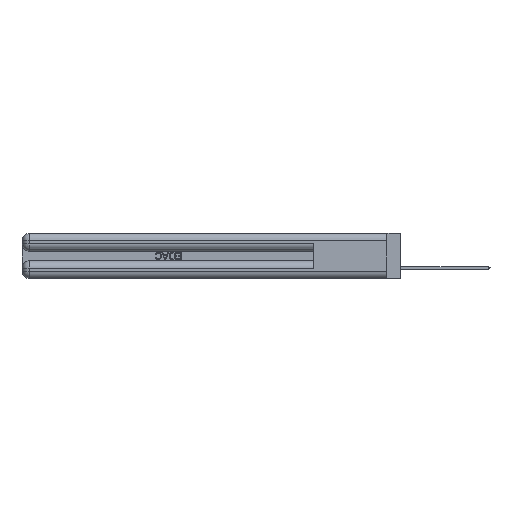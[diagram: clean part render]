
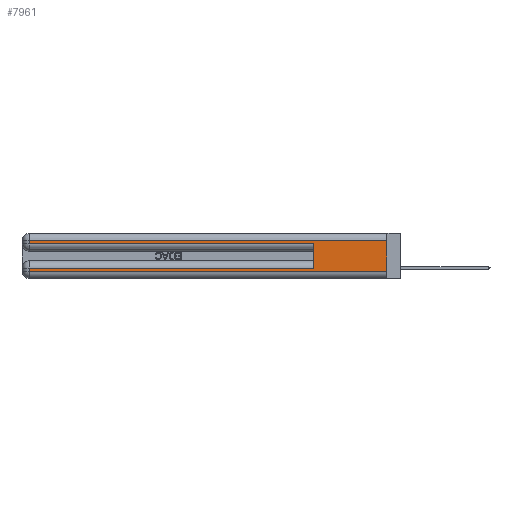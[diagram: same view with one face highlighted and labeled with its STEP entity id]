
A CAD part, left-side view. The second image highlights one B-rep face of the part: STEP entity #7961.
In plain terms, the highlighted planar face has unit normal (-1, 0, 0).
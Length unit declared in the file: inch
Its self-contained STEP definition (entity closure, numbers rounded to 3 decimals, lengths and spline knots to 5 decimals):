
#307 = VERTEX_POINT ( 'NONE', #35947 ) ;
#686 = VECTOR ( 'NONE', #15018, 39.37008 ) ;
#875 = DIRECTION ( 'NONE',  ( 0., 0., 1. ) ) ;
#906 = VERTEX_POINT ( 'NONE', #15071 ) ;
#1614 = CARTESIAN_POINT ( 'NONE',  ( 0., 0.6, 0.145 ) ) ;
#2064 = ORIENTED_EDGE ( 'NONE', *, *, #6542, .T. ) ;
#2390 = VERTEX_POINT ( 'NONE', #4002 ) ;
#2980 = CARTESIAN_POINT ( 'NONE',  ( 0., 0., 0.285 ) ) ;
#4002 = CARTESIAN_POINT ( 'NONE',  ( 0., 2.94, 0.06 ) ) ;
#6542 = EDGE_CURVE ( 'NONE', #906, #47553, #38171, .T. ) ;
#6852 = EDGE_CURVE ( 'NONE', #36797, #906, #35627, .T. ) ;
#7961 = ADVANCED_FACE ( 'NONE', ( #22028 ), #9699, .F. ) ;
#8759 = CARTESIAN_POINT ( 'NONE',  ( 0., 0., 0.37 ) ) ;
#9699 = PLANE ( 'NONE',  #32679 ) ;
#9749 = ORIENTED_EDGE ( 'NONE', *, *, #37751, .F. ) ;
#9821 = VERTEX_POINT ( 'NONE', #17732 ) ;
#11307 = ORIENTED_EDGE ( 'NONE', *, *, #6852, .T. ) ;
#11469 = CARTESIAN_POINT ( 'NONE',  ( 0., 0., 0.06 ) ) ;
#12761 = LINE ( 'NONE', #8759, #19110 ) ;
#14508 = CARTESIAN_POINT ( 'NONE',  ( 0., 0., 0.31 ) ) ;
#15018 = DIRECTION ( 'NONE',  ( 0., 0., -1. ) ) ;
#15071 = CARTESIAN_POINT ( 'NONE',  ( 0., 2.94, 0.285 ) ) ;
#15476 = VECTOR ( 'NONE', #30989, 39.37008 ) ;
#16840 = ORIENTED_EDGE ( 'NONE', *, *, #33556, .T. ) ;
#16868 = EDGE_CURVE ( 'NONE', #307, #2390, #34817, .T. ) ;
#16873 = DIRECTION ( 'NONE',  ( 0., 0., -1. ) ) ;
#16973 = ORIENTED_EDGE ( 'NONE', *, *, #19357, .T. ) ;
#17632 = EDGE_LOOP ( 'NONE', ( #40382, #16973, #11307, #2064, #9749, #35689, #32387, #16840 ) ) ;
#17732 = CARTESIAN_POINT ( 'NONE',  ( 0., 0., 0.06 ) ) ;
#17960 = CARTESIAN_POINT ( 'NONE',  ( 0., 0.6, 0.085 ) ) ;
#19110 = VECTOR ( 'NONE', #16873, 39.37008 ) ;
#19357 = EDGE_CURVE ( 'NONE', #49574, #36797, #33866, .T. ) ;
#19850 = DIRECTION ( 'NONE',  ( 0., -1., 0. ) ) ;
#20785 = CARTESIAN_POINT ( 'NONE',  ( 0., 2.94, 0.37 ) ) ;
#21712 = DIRECTION ( 'NONE',  ( 0., 0., -1. ) ) ;
#21976 = LINE ( 'NONE', #1614, #29412 ) ;
#22028 = FACE_OUTER_BOUND ( 'NONE', #17632, .T. ) ;
#22784 = VECTOR ( 'NONE', #34287, 39.37008 ) ;
#26971 = VECTOR ( 'NONE', #43122, 39.37008 ) ;
#27278 = CARTESIAN_POINT ( 'NONE',  ( 0., 0., 0.31 ) ) ;
#29412 = VECTOR ( 'NONE', #875, 39.37008 ) ;
#29976 = CARTESIAN_POINT ( 'NONE',  ( 0., 0., 0.37 ) ) ;
#30989 = DIRECTION ( 'NONE',  ( 0., -1., 0. ) ) ;
#32387 = ORIENTED_EDGE ( 'NONE', *, *, #16868, .T. ) ;
#32657 = VERTEX_POINT ( 'NONE', #17960 ) ;
#32679 = AXIS2_PLACEMENT_3D ( 'NONE', #29976, #38669, #21712 ) ;
#32737 = VECTOR ( 'NONE', #19850, 39.37008 ) ;
#33424 = LINE ( 'NONE', #50688, #22784 ) ;
#33443 = CARTESIAN_POINT ( 'NONE',  ( 0., 0.6, 0.285 ) ) ;
#33556 = EDGE_CURVE ( 'NONE', #2390, #9821, #42250, .T. ) ;
#33866 = LINE ( 'NONE', #14508, #26971 ) ;
#34287 = DIRECTION ( 'NONE',  ( 0., 1., 0. ) ) ;
#34355 = DIRECTION ( 'NONE',  ( 0., 0., -1. ) ) ;
#34817 = LINE ( 'NONE', #46950, #686 ) ;
#35239 = CARTESIAN_POINT ( 'NONE',  ( 0., 2.94, 0.31 ) ) ;
#35627 = LINE ( 'NONE', #20785, #41259 ) ;
#35689 = ORIENTED_EDGE ( 'NONE', *, *, #46441, .T. ) ;
#35947 = CARTESIAN_POINT ( 'NONE',  ( 0., 2.94, 0.085 ) ) ;
#36797 = VERTEX_POINT ( 'NONE', #35239 ) ;
#37751 = EDGE_CURVE ( 'NONE', #32657, #47553, #21976, .T. ) ;
#38171 = LINE ( 'NONE', #2980, #15476 ) ;
#38252 = EDGE_CURVE ( 'NONE', #49574, #9821, #12761, .T. ) ;
#38669 = DIRECTION ( 'NONE',  ( 1., 0., 0. ) ) ;
#40382 = ORIENTED_EDGE ( 'NONE', *, *, #38252, .F. ) ;
#41259 = VECTOR ( 'NONE', #34355, 39.37008 ) ;
#42250 = LINE ( 'NONE', #11469, #32737 ) ;
#43122 = DIRECTION ( 'NONE',  ( 0., 1., 0. ) ) ;
#46441 = EDGE_CURVE ( 'NONE', #32657, #307, #33424, .T. ) ;
#46950 = CARTESIAN_POINT ( 'NONE',  ( 0., 2.94, 0.37 ) ) ;
#47553 = VERTEX_POINT ( 'NONE', #33443 ) ;
#49574 = VERTEX_POINT ( 'NONE', #27278 ) ;
#50688 = CARTESIAN_POINT ( 'NONE',  ( 0., 0., 0.085 ) ) ;
